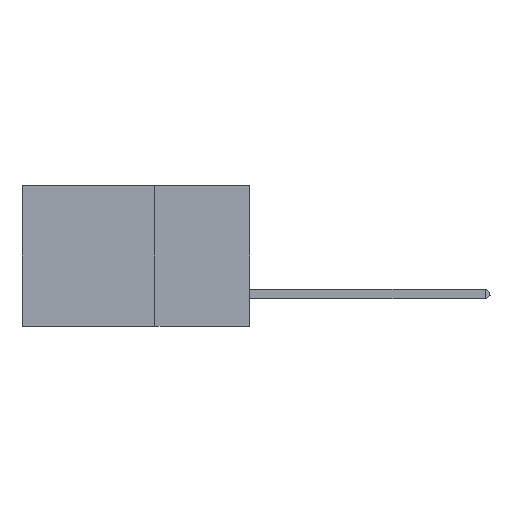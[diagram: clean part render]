
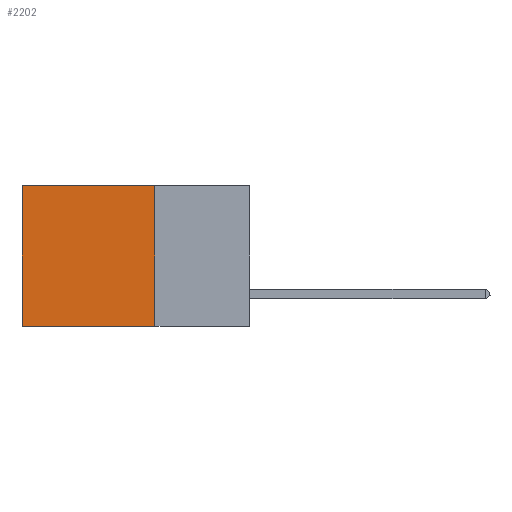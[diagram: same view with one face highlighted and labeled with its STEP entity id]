
A CAD part, left-side view. The second image highlights one B-rep face of the part: STEP entity #2202.
In plain terms, the highlighted planar face has unit normal (-1, 0, 0).
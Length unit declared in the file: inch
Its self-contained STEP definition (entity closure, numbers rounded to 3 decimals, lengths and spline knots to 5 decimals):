
#1372 = CARTESIAN_POINT ( 'NONE',  ( 0.2875, 0.25, -0.37 ) ) ;
#1797 = DIRECTION ( 'NONE',  ( 0., 1., 0. ) ) ;
#2202 = ADVANCED_FACE ( 'NONE', ( #10249 ), #31324, .F. ) ;
#5265 = DIRECTION ( 'NONE',  ( 0., 0., -1. ) ) ;
#5708 = LINE ( 'NONE', #17026, #23682 ) ;
#7979 = EDGE_CURVE ( 'NONE', #20800, #8790, #5708, .T. ) ;
#8265 = VECTOR ( 'NONE', #17104, 39.37008 ) ;
#8655 = VECTOR ( 'NONE', #1797, 39.37008 ) ;
#8790 = VERTEX_POINT ( 'NONE', #21033 ) ;
#9328 = DIRECTION ( 'NONE',  ( 0., 0., -1. ) ) ;
#10249 = FACE_OUTER_BOUND ( 'NONE', #15383, .T. ) ;
#10371 = ORIENTED_EDGE ( 'NONE', *, *, #7979, .T. ) ;
#13728 = ORIENTED_EDGE ( 'NONE', *, *, #27816, .F. ) ;
#15383 = EDGE_LOOP ( 'NONE', ( #10371, #13728, #21615, #37500 ) ) ;
#15845 = CARTESIAN_POINT ( 'NONE',  ( 0.2875, 0.25, -0.37 ) ) ;
#17026 = CARTESIAN_POINT ( 'NONE',  ( 0.2875, 0.6, 0. ) ) ;
#17104 = DIRECTION ( 'NONE',  ( 0., 1., 0. ) ) ;
#18693 = CARTESIAN_POINT ( 'NONE',  ( 0.2875, 0.6, 0. ) ) ;
#18881 = LINE ( 'NONE', #38706, #8655 ) ;
#20800 = VERTEX_POINT ( 'NONE', #18693 ) ;
#21033 = CARTESIAN_POINT ( 'NONE',  ( 0.2875, 0.6, -0.37 ) ) ;
#21615 = ORIENTED_EDGE ( 'NONE', *, *, #33185, .F. ) ;
#22374 = LINE ( 'NONE', #1372, #8265 ) ;
#23682 = VECTOR ( 'NONE', #29498, 39.37008 ) ;
#23882 = CARTESIAN_POINT ( 'NONE',  ( 0.2875, 0.25, 0. ) ) ;
#25803 = VECTOR ( 'NONE', #5265, 39.37008 ) ;
#26578 = CARTESIAN_POINT ( 'NONE',  ( 0.2875, 0.25, 0. ) ) ;
#26620 = EDGE_CURVE ( 'NONE', #27909, #20800, #18881, .T. ) ;
#27816 = EDGE_CURVE ( 'NONE', #40248, #8790, #22374, .T. ) ;
#27909 = VERTEX_POINT ( 'NONE', #26578 ) ;
#29498 = DIRECTION ( 'NONE',  ( 0., 0., -1. ) ) ;
#30921 = CARTESIAN_POINT ( 'NONE',  ( 0.2875, 0.25, 0. ) ) ;
#31324 = PLANE ( 'NONE',  #34755 ) ;
#33185 = EDGE_CURVE ( 'NONE', #27909, #40248, #34081, .T. ) ;
#34081 = LINE ( 'NONE', #23882, #25803 ) ;
#34755 = AXIS2_PLACEMENT_3D ( 'NONE', #30921, #37174, #9328 ) ;
#37174 = DIRECTION ( 'NONE',  ( 1., 0., 0. ) ) ;
#37500 = ORIENTED_EDGE ( 'NONE', *, *, #26620, .T. ) ;
#38706 = CARTESIAN_POINT ( 'NONE',  ( 0.2875, 0.25, 0. ) ) ;
#40248 = VERTEX_POINT ( 'NONE', #15845 ) ;
